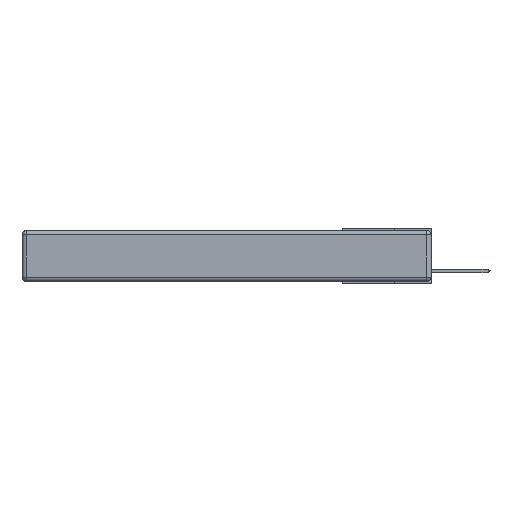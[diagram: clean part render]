
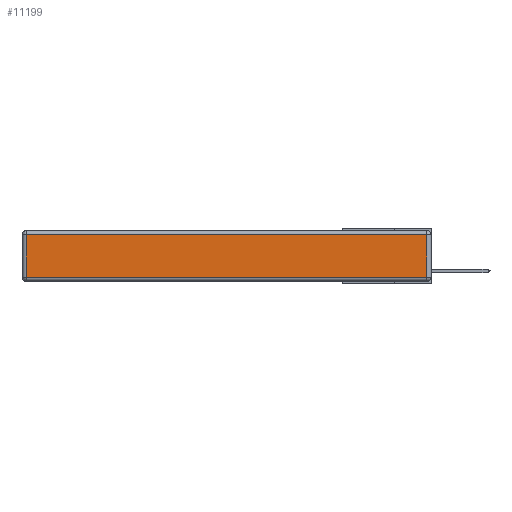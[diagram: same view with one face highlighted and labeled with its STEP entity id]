
A CAD part, left-side view. The second image highlights one B-rep face of the part: STEP entity #11199.
In plain terms, the highlighted planar face has unit normal (-1, 0, 0).
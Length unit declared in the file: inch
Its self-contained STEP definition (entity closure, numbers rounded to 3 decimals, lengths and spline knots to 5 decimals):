
#470 = AXIS2_PLACEMENT_3D ( 'NONE', #10730, #13873, #5830 ) ;
#859 = CARTESIAN_POINT ( 'NONE',  ( 0., 2.72, -0.313 ) ) ;
#1274 = DIRECTION ( 'NONE',  ( 0., 0., 1. ) ) ;
#1409 = DIRECTION ( 'NONE',  ( 0., 1., 0. ) ) ;
#1422 = CARTESIAN_POINT ( 'NONE',  ( 0., 2.72, -0.343 ) ) ;
#2023 = CARTESIAN_POINT ( 'NONE',  ( 0., 0.03, -0.313 ) ) ;
#2623 = EDGE_LOOP ( 'NONE', ( #14165, #16034, #16168, #13217 ) ) ;
#3869 = EDGE_CURVE ( 'NONE', #14853, #5867, #12154, .T. ) ;
#4690 = LINE ( 'NONE', #1422, #14944 ) ;
#4839 = DIRECTION ( 'NONE',  ( 0., -1., 0. ) ) ;
#5313 = CARTESIAN_POINT ( 'NONE',  ( 0., 0.03, -0.343 ) ) ;
#5830 = DIRECTION ( 'NONE',  ( 0., 0., 1. ) ) ;
#5867 = VERTEX_POINT ( 'NONE', #2023 ) ;
#6282 = PLANE ( 'NONE',  #470 ) ;
#6625 = EDGE_CURVE ( 'NONE', #13943, #14853, #4690, .T. ) ;
#7547 = VECTOR ( 'NONE', #1274, 39.37008 ) ;
#9454 = DIRECTION ( 'NONE',  ( 0., 0., -1. ) ) ;
#10008 = CARTESIAN_POINT ( 'NONE',  ( 0., 2.72, -0.03 ) ) ;
#10730 = CARTESIAN_POINT ( 'NONE',  ( 0., 0., -0.343 ) ) ;
#11131 = LINE ( 'NONE', #5313, #7547 ) ;
#11199 = ADVANCED_FACE ( 'NONE', ( #11490 ), #6282, .T. ) ;
#11490 = FACE_OUTER_BOUND ( 'NONE', #2623, .T. ) ;
#12154 = LINE ( 'NONE', #16967, #14020 ) ;
#12196 = CARTESIAN_POINT ( 'NONE',  ( 0., 0.03, -0.03 ) ) ;
#13217 = ORIENTED_EDGE ( 'NONE', *, *, #6625, .T. ) ;
#13873 = DIRECTION ( 'NONE',  ( -1., 0., 0. ) ) ;
#13943 = VERTEX_POINT ( 'NONE', #10008 ) ;
#14020 = VECTOR ( 'NONE', #4839, 39.37008 ) ;
#14027 = VECTOR ( 'NONE', #1409, 39.37008 ) ;
#14165 = ORIENTED_EDGE ( 'NONE', *, *, #3869, .T. ) ;
#14813 = CARTESIAN_POINT ( 'NONE',  ( 0., 2.75, -0.03 ) ) ;
#14853 = VERTEX_POINT ( 'NONE', #859 ) ;
#14944 = VECTOR ( 'NONE', #9454, 39.37008 ) ;
#14945 = VERTEX_POINT ( 'NONE', #12196 ) ;
#16034 = ORIENTED_EDGE ( 'NONE', *, *, #16480, .T. ) ;
#16168 = ORIENTED_EDGE ( 'NONE', *, *, #17289, .T. ) ;
#16480 = EDGE_CURVE ( 'NONE', #5867, #14945, #11131, .T. ) ;
#16539 = LINE ( 'NONE', #14813, #14027 ) ;
#16967 = CARTESIAN_POINT ( 'NONE',  ( 0., 0., -0.313 ) ) ;
#17289 = EDGE_CURVE ( 'NONE', #14945, #13943, #16539, .T. ) ;
